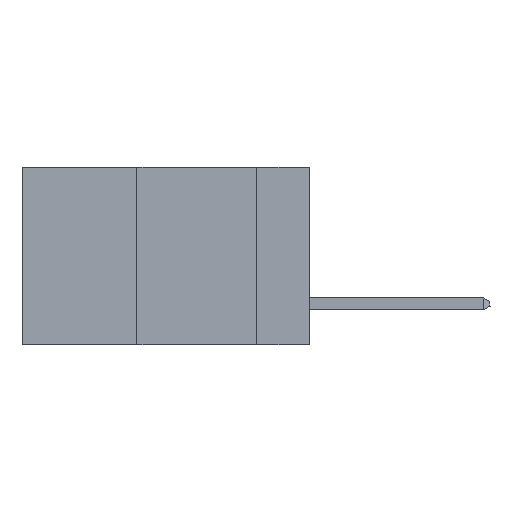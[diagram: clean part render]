
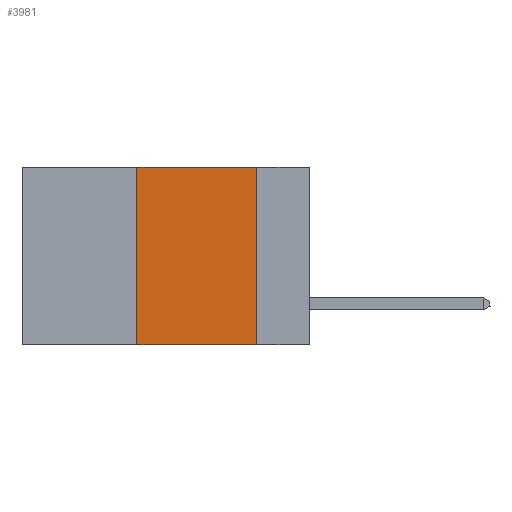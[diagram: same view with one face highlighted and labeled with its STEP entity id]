
A CAD part, left-side view. The second image highlights one B-rep face of the part: STEP entity #3981.
In plain terms, the highlighted planar face has unit normal (-1, 0, 0).
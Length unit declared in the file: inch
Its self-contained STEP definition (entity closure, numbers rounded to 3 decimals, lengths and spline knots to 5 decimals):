
#649 = AXIS2_PLACEMENT_3D ( 'NONE', #35101, #38374, #23257 ) ;
#3981 = ADVANCED_FACE ( 'NONE', ( #27962 ), #14664, .F. ) ;
#6831 = ORIENTED_EDGE ( 'NONE', *, *, #38376, .T. ) ;
#7646 = EDGE_CURVE ( 'NONE', #11129, #9265, #19594, .T. ) ;
#9265 = VERTEX_POINT ( 'NONE', #32674 ) ;
#9573 = DIRECTION ( 'NONE',  ( 0., 0., 1. ) ) ;
#10111 = LINE ( 'NONE', #15240, #11085 ) ;
#11085 = VECTOR ( 'NONE', #30877, 39.37008 ) ;
#11129 = VERTEX_POINT ( 'NONE', #30732 ) ;
#12422 = CARTESIAN_POINT ( 'NONE',  ( 0., 0.36, -0.37 ) ) ;
#13575 = ORIENTED_EDGE ( 'NONE', *, *, #7646, .F. ) ;
#13642 = EDGE_CURVE ( 'NONE', #33338, #11129, #10111, .T. ) ;
#14007 = LINE ( 'NONE', #23495, #19544 ) ;
#14664 = PLANE ( 'NONE',  #649 ) ;
#15240 = CARTESIAN_POINT ( 'NONE',  ( 0., 0.6, 0. ) ) ;
#17088 = LINE ( 'NONE', #21375, #29565 ) ;
#19544 = VECTOR ( 'NONE', #38371, 39.37008 ) ;
#19594 = LINE ( 'NONE', #37617, #28352 ) ;
#20665 = ORIENTED_EDGE ( 'NONE', *, *, #13642, .F. ) ;
#21375 = CARTESIAN_POINT ( 'NONE',  ( 0., 0.36, 0. ) ) ;
#23257 = DIRECTION ( 'NONE',  ( 0., 0., -1. ) ) ;
#23495 = CARTESIAN_POINT ( 'NONE',  ( 0., 0.6, -0.37 ) ) ;
#26899 = ORIENTED_EDGE ( 'NONE', *, *, #27643, .F. ) ;
#27643 = EDGE_CURVE ( 'NONE', #33087, #33338, #17088, .T. ) ;
#27962 = FACE_OUTER_BOUND ( 'NONE', #32117, .T. ) ;
#28352 = VECTOR ( 'NONE', #32480, 39.37008 ) ;
#28792 = CARTESIAN_POINT ( 'NONE',  ( 0., 0.36, 0. ) ) ;
#29565 = VECTOR ( 'NONE', #9573, 39.37008 ) ;
#30732 = CARTESIAN_POINT ( 'NONE',  ( 0., 0.11, 0. ) ) ;
#30877 = DIRECTION ( 'NONE',  ( 0., -1., 0. ) ) ;
#32117 = EDGE_LOOP ( 'NONE', ( #13575, #20665, #26899, #6831 ) ) ;
#32480 = DIRECTION ( 'NONE',  ( 0., 0., -1. ) ) ;
#32674 = CARTESIAN_POINT ( 'NONE',  ( 0., 0.11, -0.37 ) ) ;
#33087 = VERTEX_POINT ( 'NONE', #12422 ) ;
#33338 = VERTEX_POINT ( 'NONE', #28792 ) ;
#35101 = CARTESIAN_POINT ( 'NONE',  ( 0., 0.6, 0. ) ) ;
#37617 = CARTESIAN_POINT ( 'NONE',  ( 0., 0.11, 0. ) ) ;
#38371 = DIRECTION ( 'NONE',  ( 0., -1., 0. ) ) ;
#38374 = DIRECTION ( 'NONE',  ( 1., 0., 0. ) ) ;
#38376 = EDGE_CURVE ( 'NONE', #33087, #9265, #14007, .T. ) ;
